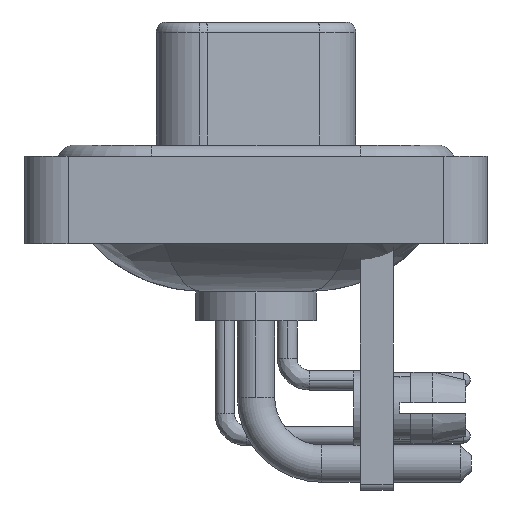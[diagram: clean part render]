
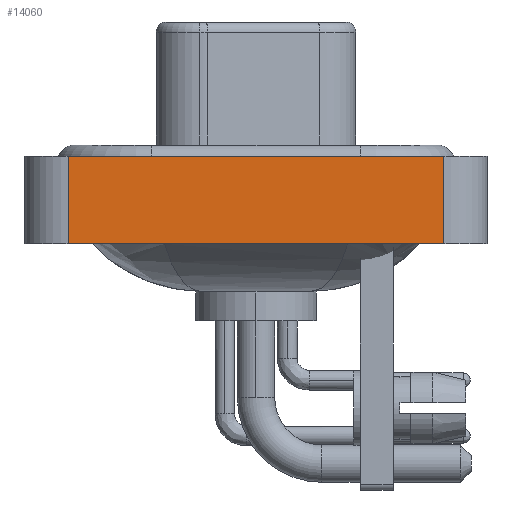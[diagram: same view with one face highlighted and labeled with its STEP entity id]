
A CAD part, left-side view. The second image highlights one B-rep face of the part: STEP entity #14060.
In plain terms, the highlighted planar face has unit normal (-1, 0, 0).
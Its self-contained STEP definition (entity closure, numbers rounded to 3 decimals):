
#1170 = VERTEX_POINT ( 'NONE', #9337 ) ;
#1388 = DIRECTION ( 'NONE',  ( -1., 0., 0. ) ) ;
#1810 = CARTESIAN_POINT ( 'NONE',  ( -7.35, -8.55, -3.6 ) ) ;
#3219 = VECTOR ( 'NONE', #26990, 1000. ) ;
#4254 = CARTESIAN_POINT ( 'NONE',  ( -7.35, -8.55, -3.6 ) ) ;
#4274 = DIRECTION ( 'NONE',  ( 0., -1., 0. ) ) ;
#5606 = DIRECTION ( 'NONE',  ( 0., 0., 1. ) ) ;
#6008 = VECTOR ( 'NONE', #5606, 1000. ) ;
#6272 = CARTESIAN_POINT ( 'NONE',  ( -7.35, -8.55, 0.4 ) ) ;
#6564 = CARTESIAN_POINT ( 'NONE',  ( -7.35, 8.55, -3.6 ) ) ;
#7081 = VECTOR ( 'NONE', #4274, 1000. ) ;
#7105 = VECTOR ( 'NONE', #20225, 1000. ) ;
#7159 = ORIENTED_EDGE ( 'NONE', *, *, #27145, .T. ) ;
#8460 = LINE ( 'NONE', #20322, #7081 ) ;
#9337 = CARTESIAN_POINT ( 'NONE',  ( -7.35, 8.55, -3.6 ) ) ;
#10650 = EDGE_CURVE ( 'NONE', #1170, #29382, #22648, .T. ) ;
#12511 = CARTESIAN_POINT ( 'NONE',  ( -7.35, -8.55, -3.6 ) ) ;
#13599 = ORIENTED_EDGE ( 'NONE', *, *, #10650, .T. ) ;
#14060 = ADVANCED_FACE ( 'NONE', ( #15660 ), #24774, .T. ) ;
#14418 = EDGE_CURVE ( 'NONE', #1170, #27816, #26801, .T. ) ;
#14467 = VERTEX_POINT ( 'NONE', #6272 ) ;
#15660 = FACE_OUTER_BOUND ( 'NONE', #26224, .T. ) ;
#16360 = CARTESIAN_POINT ( 'NONE',  ( -7.35, 8.55, 0.4 ) ) ;
#17163 = LINE ( 'NONE', #12511, #6008 ) ;
#20225 = DIRECTION ( 'NONE',  ( 0., 0., 1. ) ) ;
#20322 = CARTESIAN_POINT ( 'NONE',  ( -7.35, -8.55, 0.4 ) ) ;
#21111 = AXIS2_PLACEMENT_3D ( 'NONE', #4254, #1388, #28808 ) ;
#22648 = LINE ( 'NONE', #1810, #3219 ) ;
#23802 = EDGE_CURVE ( 'NONE', #27816, #14467, #8460, .T. ) ;
#24774 = PLANE ( 'NONE',  #21111 ) ;
#25546 = ORIENTED_EDGE ( 'NONE', *, *, #14418, .F. ) ;
#26224 = EDGE_LOOP ( 'NONE', ( #7159, #28107, #25546, #13599 ) ) ;
#26801 = LINE ( 'NONE', #6564, #7105 ) ;
#26990 = DIRECTION ( 'NONE',  ( 0., -1., 0. ) ) ;
#27145 = EDGE_CURVE ( 'NONE', #29382, #14467, #17163, .T. ) ;
#27816 = VERTEX_POINT ( 'NONE', #16360 ) ;
#28107 = ORIENTED_EDGE ( 'NONE', *, *, #23802, .F. ) ;
#28751 = CARTESIAN_POINT ( 'NONE',  ( -7.35, -8.55, -3.6 ) ) ;
#28808 = DIRECTION ( 'NONE',  ( 0., 0., 1. ) ) ;
#29382 = VERTEX_POINT ( 'NONE', #28751 ) ;
